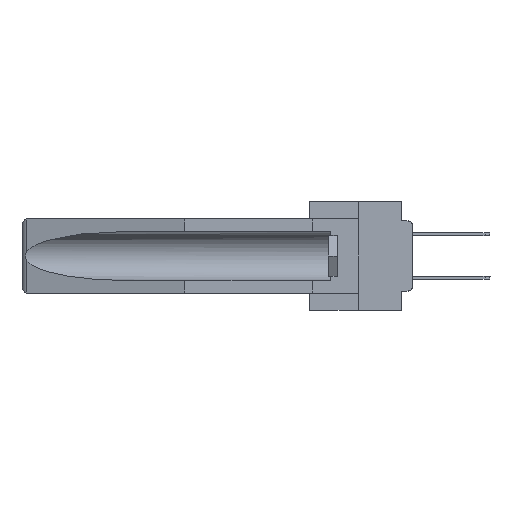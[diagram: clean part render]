
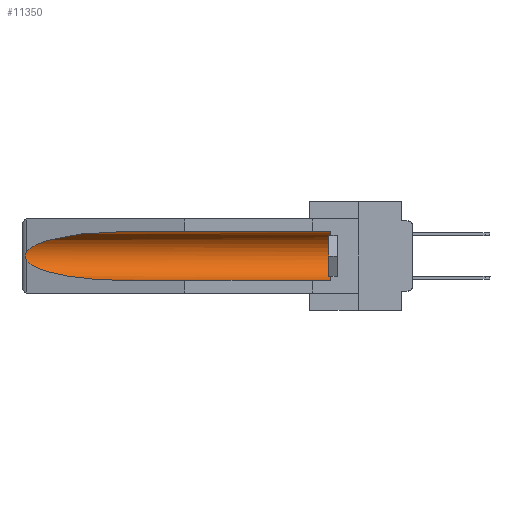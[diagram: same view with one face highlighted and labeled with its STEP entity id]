
A CAD part, left-side view. The second image highlights one B-rep face of the part: STEP entity #11350.
In plain terms, the highlighted cylindrical face has radius 2.857 mm (diameter 5.715 mm), a partial arc.
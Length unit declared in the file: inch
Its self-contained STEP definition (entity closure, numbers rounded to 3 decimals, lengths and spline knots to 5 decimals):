
#53 = DIRECTION ( 'NONE',  ( 0., 0., 1. ) ) ;
#346 = AXIS2_PLACEMENT_3D ( 'NONE', #27302, #21178, #53 ) ;
#985 = CARTESIAN_POINT ( 'NONE',  ( 0.26597, 1.52961, -0.15275 ) ) ;
#1106 = VERTEX_POINT ( 'NONE', #7148 ) ;
#1957 = DIRECTION ( 'NONE',  ( 0., 1., 0. ) ) ;
#2543 = EDGE_CURVE ( 'NONE', #5349, #7713, #29985, .T. ) ;
#3513 = EDGE_CURVE ( 'NONE', #23663, #5349, #10436, .T. ) ;
#4222 = EDGE_CURVE ( 'NONE', #20639, #1106, #32655, .T. ) ;
#4939 = CARTESIAN_POINT ( 'NONE',  ( 0.155, -0.30754, -0.284 ) ) ;
#5349 = VERTEX_POINT ( 'NONE', #29875 ) ;
#5470 = CARTESIAN_POINT ( 'NONE',  ( 0.25451, 1.48313, -0.09465 ) ) ;
#5604 = ORIENTED_EDGE ( 'NONE', *, *, #4222, .T. ) ;
#7148 = CARTESIAN_POINT ( 'NONE',  ( 0.26537, 1.52718, -0.19328 ) ) ;
#7713 = VERTEX_POINT ( 'NONE', #38523 ) ;
#8073 = ORIENTED_EDGE ( 'NONE', *, *, #19041, .T. ) ;
#8216 = EDGE_CURVE ( 'NONE', #23663, #35159, #19943, .T. ) ;
#8392 = DIRECTION ( 'NONE',  ( 0., 1., 0. ) ) ;
#8787 = CARTESIAN_POINT ( 'NONE',  ( 0.21114, 1.30732, -0.284 ) ) ;
#9037 = DIRECTION ( 'NONE',  ( 0., 1., 0. ) ) ;
#9349 =( BOUNDED_CURVE ( )  B_SPLINE_CURVE ( 3, ( #14535, #32532, #5470, #26219 ),
 .UNSPECIFIED., .F., .F. ) 
 B_SPLINE_CURVE_WITH_KNOTS ( ( 4, 4 ),
 ( 4.71239, 6.08839 ),
 .UNSPECIFIED. ) 
 CURVE ( )  GEOMETRIC_REPRESENTATION_ITEM ( )  RATIONAL_B_SPLINE_CURVE ( ( 1., 0.848, 0.848, 1. ) ) 
 REPRESENTATION_ITEM ( '' )  );
#10068 = CARTESIAN_POINT ( 'NONE',  ( 0.2675, 1.53308, -0.16763 ) ) ;
#10436 = CIRCLE ( 'NONE', #346, 0.1125 ) ;
#11153 = FACE_OUTER_BOUND ( 'NONE', #32545, .T. ) ;
#11350 = ADVANCED_FACE ( 'NONE', ( #11153 ), #35280, .F. ) ;
#12135 = CARTESIAN_POINT ( 'NONE',  ( 0.26537, 1.52718, -0.14972 ) ) ;
#13024 = CARTESIAN_POINT ( 'NONE',  ( 0.26654, 1.53092, -0.15636 ) ) ;
#14535 = CARTESIAN_POINT ( 'NONE',  ( 0.155, 1.07973, -0.059 ) ) ;
#16196 = CARTESIAN_POINT ( 'NONE',  ( 0.2675, 1.53308, -0.17534 ) ) ;
#17287 = CARTESIAN_POINT ( 'NONE',  ( 0.155, -0.30754, -0.1715 ) ) ;
#18205 = VECTOR ( 'NONE', #1957, 39.37008 ) ;
#19041 = EDGE_CURVE ( 'NONE', #7713, #20639, #9349, .T. ) ;
#19943 = LINE ( 'NONE', #4939, #18205 ) ;
#20133 = CARTESIAN_POINT ( 'NONE',  ( 0.26537, 1.52718, -0.19328 ) ) ;
#20639 = VERTEX_POINT ( 'NONE', #12135 ) ;
#20803 = CARTESIAN_POINT ( 'NONE',  ( 0.155, 1.07973, -0.284 ) ) ;
#21178 = DIRECTION ( 'NONE',  ( 0., -1., 0. ) ) ;
#21191 = ORIENTED_EDGE ( 'NONE', *, *, #31970, .T. ) ;
#22036 = ORIENTED_EDGE ( 'NONE', *, *, #2543, .T. ) ;
#22893 = CARTESIAN_POINT ( 'NONE',  ( 0.155, -0.30754, -0.059 ) ) ;
#23459 = AXIS2_PLACEMENT_3D ( 'NONE', #17287, #8392, #23586 ) ;
#23586 = DIRECTION ( 'NONE',  ( 0., 0., 1. ) ) ;
#23663 = VERTEX_POINT ( 'NONE', #28654 ) ;
#25085 = CARTESIAN_POINT ( 'NONE',  ( 0.2673, 1.5327, -0.16383 ) ) ;
#25278 = CARTESIAN_POINT ( 'NONE',  ( 0.26655, 1.53094, -0.18657 ) ) ;
#26219 = CARTESIAN_POINT ( 'NONE',  ( 0.26537, 1.52718, -0.14972 ) ) ;
#26406 = ORIENTED_EDGE ( 'NONE', *, *, #8216, .F. ) ;
#27302 = CARTESIAN_POINT ( 'NONE',  ( 0.155, 0.126, -0.1715 ) ) ;
#28063 = CARTESIAN_POINT ( 'NONE',  ( 0.26537, 1.52718, -0.14972 ) ) ;
#28256 = CARTESIAN_POINT ( 'NONE',  ( 0.2673, 1.53269, -0.17917 ) ) ;
#28654 = CARTESIAN_POINT ( 'NONE',  ( 0.155, 0.126, -0.284 ) ) ;
#29875 = CARTESIAN_POINT ( 'NONE',  ( 0.155, 0.126, -0.059 ) ) ;
#29985 = LINE ( 'NONE', #22893, #32230 ) ;
#31924 = ORIENTED_EDGE ( 'NONE', *, *, #3513, .T. ) ;
#31970 = EDGE_CURVE ( 'NONE', #1106, #35159, #33589, .T. ) ;
#32230 = VECTOR ( 'NONE', #9037, 39.37008 ) ;
#32508 = CARTESIAN_POINT ( 'NONE',  ( 0.26537, 1.52718, -0.19328 ) ) ;
#32532 = CARTESIAN_POINT ( 'NONE',  ( 0.21114, 1.30732, -0.059 ) ) ;
#32545 = EDGE_LOOP ( 'NONE', ( #8073, #5604, #21191, #26406, #31924, #22036 ) ) ;
#32655 = B_SPLINE_CURVE_WITH_KNOTS ( 'NONE', 3,
 ( #28063, #985, #13024, #25085, #10068, #16196, #28256, #25278, #37342, #20133 ),
 .UNSPECIFIED., .F., .F.,
 ( 4, 2, 2, 2, 4 ),
 ( 0., 0.00029, 0.00058, 0.00087, 0.00117 ),
 .UNSPECIFIED. ) ;
#33589 =( BOUNDED_CURVE ( )  B_SPLINE_CURVE ( 3, ( #32508, #38631, #8787, #20803 ),
 .UNSPECIFIED., .F., .F. ) 
 B_SPLINE_CURVE_WITH_KNOTS ( ( 4, 4 ),
 ( 0.1948, 1.5708 ),
 .UNSPECIFIED. ) 
 CURVE ( )  GEOMETRIC_REPRESENTATION_ITEM ( )  RATIONAL_B_SPLINE_CURVE ( ( 1., 0.848, 0.848, 1. ) ) 
 REPRESENTATION_ITEM ( '' )  );
#34641 = CARTESIAN_POINT ( 'NONE',  ( 0.155, 1.07973, -0.284 ) ) ;
#35159 = VERTEX_POINT ( 'NONE', #34641 ) ;
#35280 = CYLINDRICAL_SURFACE ( 'NONE', #23459, 0.1125 ) ;
#37342 = CARTESIAN_POINT ( 'NONE',  ( 0.26597, 1.5296, -0.19026 ) ) ;
#38523 = CARTESIAN_POINT ( 'NONE',  ( 0.155, 1.07973, -0.059 ) ) ;
#38631 = CARTESIAN_POINT ( 'NONE',  ( 0.25451, 1.48313, -0.24835 ) ) ;
